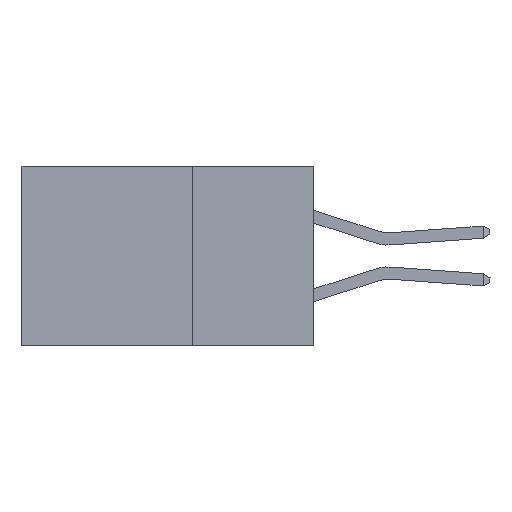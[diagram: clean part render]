
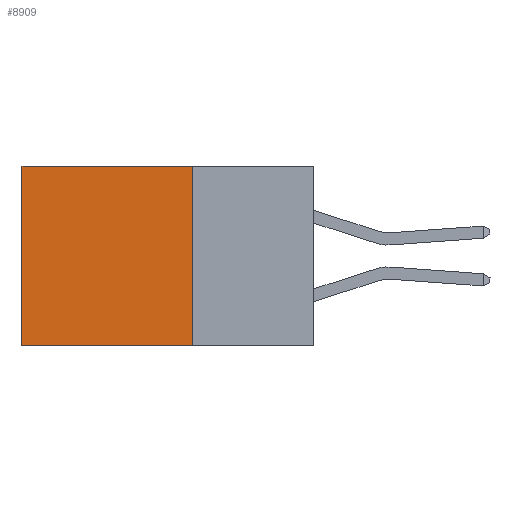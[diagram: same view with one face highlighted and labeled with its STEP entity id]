
A CAD part, left-side view. The second image highlights one B-rep face of the part: STEP entity #8909.
In plain terms, the highlighted planar face has unit normal (-1, 0, 0).
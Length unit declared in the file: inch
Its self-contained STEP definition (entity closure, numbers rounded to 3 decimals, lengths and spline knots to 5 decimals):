
#375 = EDGE_CURVE ( 'NONE', #23838, #18163, #7458, .T. ) ;
#3170 = DIRECTION ( 'NONE',  ( 0., 0., -1. ) ) ;
#3517 = CARTESIAN_POINT ( 'NONE',  ( 0.2875, 0.6, 0. ) ) ;
#4807 = ORIENTED_EDGE ( 'NONE', *, *, #16507, .T. ) ;
#5514 = PLANE ( 'NONE',  #9032 ) ;
#5703 = DIRECTION ( 'NONE',  ( 0., 1., 0. ) ) ;
#5860 = DIRECTION ( 'NONE',  ( 1., 0., 0. ) ) ;
#7458 = LINE ( 'NONE', #19477, #9568 ) ;
#8909 = ADVANCED_FACE ( 'NONE', ( #11122 ), #5514, .F. ) ;
#8969 = CARTESIAN_POINT ( 'NONE',  ( 0.2875, 0.25, 0. ) ) ;
#9032 = AXIS2_PLACEMENT_3D ( 'NONE', #30087, #5860, #3170 ) ;
#9568 = VECTOR ( 'NONE', #5703, 39.37008 ) ;
#9826 = ORIENTED_EDGE ( 'NONE', *, *, #29405, .T. ) ;
#11122 = FACE_OUTER_BOUND ( 'NONE', #18405, .T. ) ;
#11286 = DIRECTION ( 'NONE',  ( 0., 0., -1. ) ) ;
#12011 = CARTESIAN_POINT ( 'NONE',  ( 0.2875, 0.25, -0.37 ) ) ;
#13227 = VECTOR ( 'NONE', #11286, 39.37008 ) ;
#14166 = DIRECTION ( 'NONE',  ( 0., 1., 0. ) ) ;
#14857 = VECTOR ( 'NONE', #34075, 39.37008 ) ;
#16507 = EDGE_CURVE ( 'NONE', #32197, #18163, #25893, .T. ) ;
#17086 = EDGE_CURVE ( 'NONE', #31993, #23838, #19083, .T. ) ;
#18163 = VERTEX_POINT ( 'NONE', #31226 ) ;
#18405 = EDGE_LOOP ( 'NONE', ( #4807, #20170, #28938, #9826 ) ) ;
#19083 = LINE ( 'NONE', #28860, #14857 ) ;
#19477 = CARTESIAN_POINT ( 'NONE',  ( 0.2875, 0.25, -0.37 ) ) ;
#20170 = ORIENTED_EDGE ( 'NONE', *, *, #375, .F. ) ;
#22817 = VECTOR ( 'NONE', #14166, 39.37008 ) ;
#23838 = VERTEX_POINT ( 'NONE', #12011 ) ;
#24271 = CARTESIAN_POINT ( 'NONE',  ( 0.2875, 0.6, 0. ) ) ;
#25893 = LINE ( 'NONE', #3517, #13227 ) ;
#28860 = CARTESIAN_POINT ( 'NONE',  ( 0.2875, 0.25, 0. ) ) ;
#28938 = ORIENTED_EDGE ( 'NONE', *, *, #17086, .F. ) ;
#29041 = CARTESIAN_POINT ( 'NONE',  ( 0.2875, 0.25, 0. ) ) ;
#29193 = LINE ( 'NONE', #8969, #22817 ) ;
#29405 = EDGE_CURVE ( 'NONE', #31993, #32197, #29193, .T. ) ;
#30087 = CARTESIAN_POINT ( 'NONE',  ( 0.2875, 0.25, 0. ) ) ;
#31226 = CARTESIAN_POINT ( 'NONE',  ( 0.2875, 0.6, -0.37 ) ) ;
#31993 = VERTEX_POINT ( 'NONE', #29041 ) ;
#32197 = VERTEX_POINT ( 'NONE', #24271 ) ;
#34075 = DIRECTION ( 'NONE',  ( 0., 0., -1. ) ) ;
